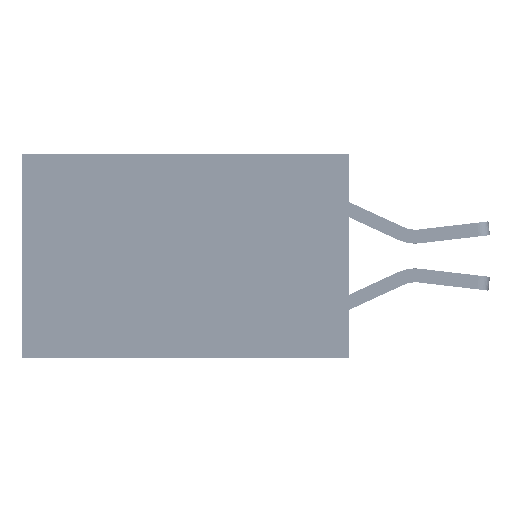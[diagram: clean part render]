
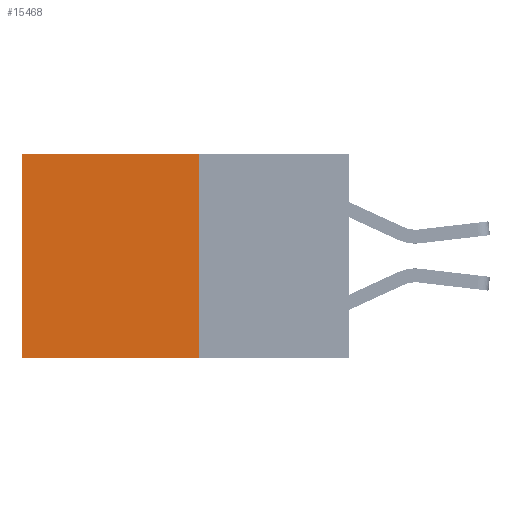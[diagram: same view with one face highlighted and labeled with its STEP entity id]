
A CAD part, left-side view. The second image highlights one B-rep face of the part: STEP entity #15468.
In plain terms, the highlighted planar face has unit normal (-1, 0, 0).
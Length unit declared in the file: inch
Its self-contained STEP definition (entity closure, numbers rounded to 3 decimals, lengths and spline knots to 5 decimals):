
#40 = LINE ( 'NONE', #25065, #27284 ) ;
#1085 = CARTESIAN_POINT ( 'NONE',  ( 0.277, 0.59, -0.37 ) ) ;
#1315 = AXIS2_PLACEMENT_3D ( 'NONE', #24447, #32295, #16668 ) ;
#2706 = EDGE_LOOP ( 'NONE', ( #12945, #5714, #8513, #16974 ) ) ;
#2831 = VERTEX_POINT ( 'NONE', #23420 ) ;
#3681 = EDGE_CURVE ( 'NONE', #9610, #12371, #18434, .T. ) ;
#5714 = ORIENTED_EDGE ( 'NONE', *, *, #3681, .F. ) ;
#6288 = VECTOR ( 'NONE', #21629, 39.37008 ) ;
#6323 = DIRECTION ( 'NONE',  ( 0., 0., -1. ) ) ;
#8457 = CARTESIAN_POINT ( 'NONE',  ( 0.277, 0.27, -0.37 ) ) ;
#8513 = ORIENTED_EDGE ( 'NONE', *, *, #32015, .F. ) ;
#9610 = VERTEX_POINT ( 'NONE', #13757 ) ;
#12371 = VERTEX_POINT ( 'NONE', #16456 ) ;
#12945 = ORIENTED_EDGE ( 'NONE', *, *, #21823, .T. ) ;
#13757 = CARTESIAN_POINT ( 'NONE',  ( 0.277, 0.27, -0.37 ) ) ;
#13992 = PLANE ( 'NONE',  #1315 ) ;
#14688 = CARTESIAN_POINT ( 'NONE',  ( 0.277, 0.59, 0. ) ) ;
#15468 = ADVANCED_FACE ( 'NONE', ( #30292 ), #13992, .F. ) ;
#16456 = CARTESIAN_POINT ( 'NONE',  ( 0.277, 0.59, -0.37 ) ) ;
#16668 = DIRECTION ( 'NONE',  ( 0., 0., -1. ) ) ;
#16974 = ORIENTED_EDGE ( 'NONE', *, *, #31542, .T. ) ;
#17301 = DIRECTION ( 'NONE',  ( 0., 1., 0. ) ) ;
#18434 = LINE ( 'NONE', #31056, #32301 ) ;
#21629 = DIRECTION ( 'NONE',  ( 0., 0., -1. ) ) ;
#21823 = EDGE_CURVE ( 'NONE', #23189, #12371, #26891, .T. ) ;
#23189 = VERTEX_POINT ( 'NONE', #14688 ) ;
#23420 = CARTESIAN_POINT ( 'NONE',  ( 0.277, 0.27, 0. ) ) ;
#24447 = CARTESIAN_POINT ( 'NONE',  ( 0.277, 0.27, -0.37 ) ) ;
#25065 = CARTESIAN_POINT ( 'NONE',  ( 0.277, 0.27, 0. ) ) ;
#26448 = LINE ( 'NONE', #8457, #6288 ) ;
#26891 = LINE ( 'NONE', #1085, #32984 ) ;
#27284 = VECTOR ( 'NONE', #17301, 39.37008 ) ;
#30292 = FACE_OUTER_BOUND ( 'NONE', #2706, .T. ) ;
#31014 = DIRECTION ( 'NONE',  ( 0., 1., 0. ) ) ;
#31056 = CARTESIAN_POINT ( 'NONE',  ( 0.277, 0.27, -0.37 ) ) ;
#31542 = EDGE_CURVE ( 'NONE', #2831, #23189, #40, .T. ) ;
#32015 = EDGE_CURVE ( 'NONE', #2831, #9610, #26448, .T. ) ;
#32295 = DIRECTION ( 'NONE',  ( 1., 0., 0. ) ) ;
#32301 = VECTOR ( 'NONE', #31014, 39.37008 ) ;
#32984 = VECTOR ( 'NONE', #6323, 39.37008 ) ;
